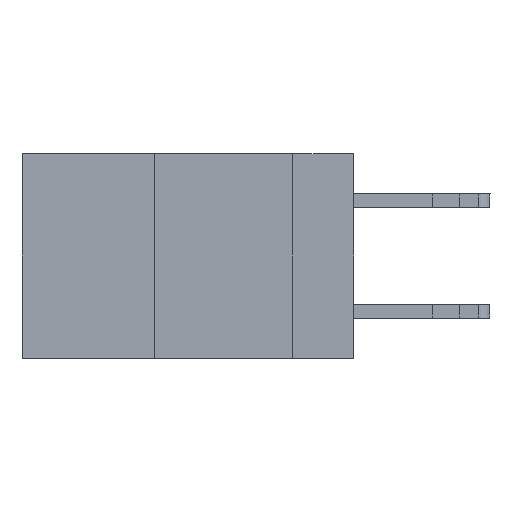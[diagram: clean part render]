
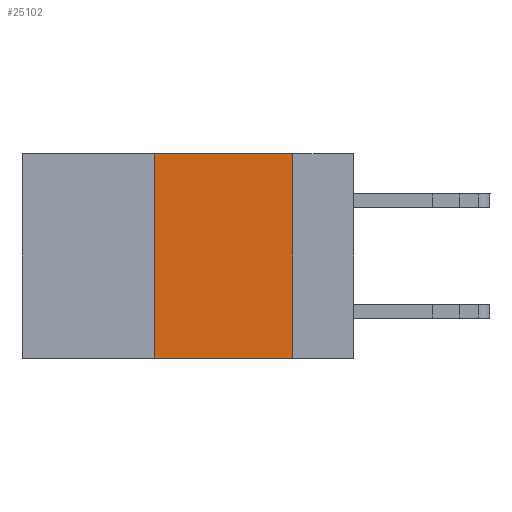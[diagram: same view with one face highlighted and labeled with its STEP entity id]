
A CAD part, left-side view. The second image highlights one B-rep face of the part: STEP entity #25102.
In plain terms, the highlighted planar face has unit normal (-1, 0, 0).
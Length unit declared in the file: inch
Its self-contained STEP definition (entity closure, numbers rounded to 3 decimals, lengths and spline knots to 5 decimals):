
#646 = CARTESIAN_POINT ( 'NONE',  ( 0., 0.36, -0.37 ) ) ;
#848 = EDGE_CURVE ( 'NONE', #4837, #5999, #24206, .T. ) ;
#1968 = CARTESIAN_POINT ( 'NONE',  ( 0., 0.36, 0. ) ) ;
#2885 = ORIENTED_EDGE ( 'NONE', *, *, #848, .T. ) ;
#4837 = VERTEX_POINT ( 'NONE', #646 ) ;
#5999 = VERTEX_POINT ( 'NONE', #7446 ) ;
#6249 = LINE ( 'NONE', #22141, #20797 ) ;
#7446 = CARTESIAN_POINT ( 'NONE',  ( 0., 0.11, -0.37 ) ) ;
#8985 = LINE ( 'NONE', #27816, #33573 ) ;
#9849 = ORIENTED_EDGE ( 'NONE', *, *, #29245, .F. ) ;
#10114 = PLANE ( 'NONE',  #27695 ) ;
#11241 = ORIENTED_EDGE ( 'NONE', *, *, #13980, .F. ) ;
#12103 = DIRECTION ( 'NONE',  ( 0., 0., -1. ) ) ;
#12180 = VECTOR ( 'NONE', #27725, 39.37008 ) ;
#13261 = VERTEX_POINT ( 'NONE', #27082 ) ;
#13980 = EDGE_CURVE ( 'NONE', #4837, #27049, #33407, .T. ) ;
#16454 = DIRECTION ( 'NONE',  ( 0., -1., 0. ) ) ;
#19309 = EDGE_CURVE ( 'NONE', #27049, #13261, #6249, .T. ) ;
#20133 = DIRECTION ( 'NONE',  ( 0., 0., -1. ) ) ;
#20797 = VECTOR ( 'NONE', #16454, 39.37008 ) ;
#20817 = DIRECTION ( 'NONE',  ( 1., 0., 0. ) ) ;
#22141 = CARTESIAN_POINT ( 'NONE',  ( 0., 0.6, 0. ) ) ;
#24206 = LINE ( 'NONE', #29410, #26732 ) ;
#25102 = ADVANCED_FACE ( 'NONE', ( #33258 ), #10114, .F. ) ;
#25998 = CARTESIAN_POINT ( 'NONE',  ( 0., 0.6, 0. ) ) ;
#26641 = DIRECTION ( 'NONE',  ( 0., -1., 0. ) ) ;
#26732 = VECTOR ( 'NONE', #26641, 39.37008 ) ;
#27049 = VERTEX_POINT ( 'NONE', #32507 ) ;
#27082 = CARTESIAN_POINT ( 'NONE',  ( 0., 0.11, 0. ) ) ;
#27695 = AXIS2_PLACEMENT_3D ( 'NONE', #25998, #20817, #20133 ) ;
#27725 = DIRECTION ( 'NONE',  ( 0., 0., 1. ) ) ;
#27816 = CARTESIAN_POINT ( 'NONE',  ( 0., 0.11, 0. ) ) ;
#29245 = EDGE_CURVE ( 'NONE', #13261, #5999, #8985, .T. ) ;
#29410 = CARTESIAN_POINT ( 'NONE',  ( 0., 0.6, -0.37 ) ) ;
#30289 = EDGE_LOOP ( 'NONE', ( #9849, #30664, #11241, #2885 ) ) ;
#30664 = ORIENTED_EDGE ( 'NONE', *, *, #19309, .F. ) ;
#32507 = CARTESIAN_POINT ( 'NONE',  ( 0., 0.36, 0. ) ) ;
#33258 = FACE_OUTER_BOUND ( 'NONE', #30289, .T. ) ;
#33407 = LINE ( 'NONE', #1968, #12180 ) ;
#33573 = VECTOR ( 'NONE', #12103, 39.37008 ) ;
